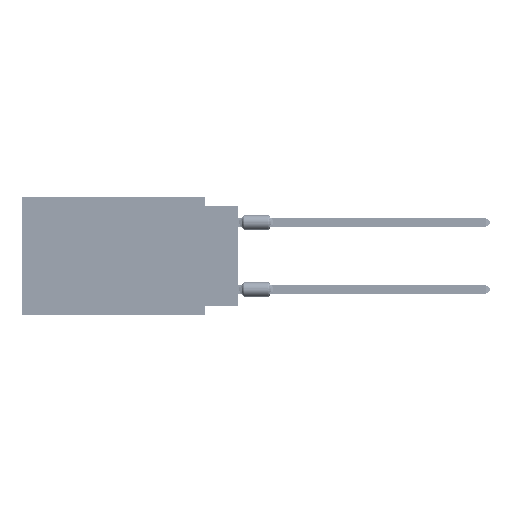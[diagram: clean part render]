
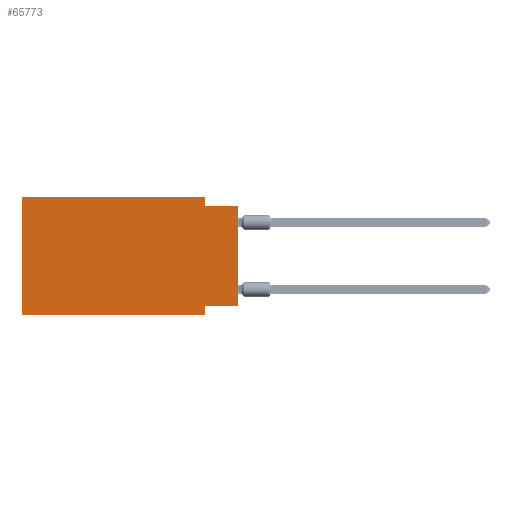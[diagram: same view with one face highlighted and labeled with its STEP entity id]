
A CAD part, left-side view. The second image highlights one B-rep face of the part: STEP entity #65773.
In plain terms, the highlighted planar face has unit normal (-1, 0, 0).
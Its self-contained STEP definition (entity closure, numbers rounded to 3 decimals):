
#11 = CARTESIAN_POINT ( 'NONE',  ( 0., 0., -0.635 ) ) ;
#284 = VERTEX_POINT ( 'NONE', #22249 ) ;
#1347 = DIRECTION ( 'NONE',  ( 1., 0., 0. ) ) ;
#1733 = LINE ( 'NONE', #33577, #5530 ) ;
#3929 = CARTESIAN_POINT ( 'NONE',  ( 0., 2.54, -0.635 ) ) ;
#5530 = VECTOR ( 'NONE', #74538, 1000. ) ;
#5900 = ORIENTED_EDGE ( 'NONE', *, *, #55489, .T. ) ;
#6079 = ORIENTED_EDGE ( 'NONE', *, *, #68950, .F. ) ;
#7489 = VECTOR ( 'NONE', #74238, 1000. ) ;
#7572 = LINE ( 'NONE', #34146, #7489 ) ;
#8371 = LINE ( 'NONE', #22303, #59228 ) ;
#11328 = VECTOR ( 'NONE', #56638, 1000. ) ;
#14348 = VERTEX_POINT ( 'NONE', #56754 ) ;
#15757 = DIRECTION ( 'NONE',  ( 0., -1., 0. ) ) ;
#15805 = CARTESIAN_POINT ( 'NONE',  ( 0., 16.383, 0. ) ) ;
#18344 = LINE ( 'NONE', #57554, #56484 ) ;
#18844 = EDGE_CURVE ( 'NONE', #57992, #76201, #7572, .T. ) ;
#20351 = VECTOR ( 'NONE', #59810, 1000. ) ;
#22249 = CARTESIAN_POINT ( 'NONE',  ( 0., 16.383, 0. ) ) ;
#22303 = CARTESIAN_POINT ( 'NONE',  ( 0., 16.383, 0. ) ) ;
#23098 = LINE ( 'NONE', #49666, #11328 ) ;
#23633 = LINE ( 'NONE', #15805, #83268 ) ;
#24822 = EDGE_CURVE ( 'NONE', #14348, #79552, #18344, .T. ) ;
#27155 = EDGE_CURVE ( 'NONE', #57992, #284, #23633, .T. ) ;
#32731 = EDGE_CURVE ( 'NONE', #65692, #35897, #23098, .T. ) ;
#33174 = FACE_OUTER_BOUND ( 'NONE', #43064, .T. ) ;
#33577 = CARTESIAN_POINT ( 'NONE',  ( 0., 2.54, -8.89 ) ) ;
#34146 = CARTESIAN_POINT ( 'NONE',  ( 0., 16.383, -8.89 ) ) ;
#35132 = ORIENTED_EDGE ( 'NONE', *, *, #53036, .F. ) ;
#35801 = ORIENTED_EDGE ( 'NONE', *, *, #59684, .F. ) ;
#35838 = DIRECTION ( 'NONE',  ( 0., 0., 1. ) ) ;
#35897 = VERTEX_POINT ( 'NONE', #3929 ) ;
#36611 = CARTESIAN_POINT ( 'NONE',  ( 0., 2.54, -8.255 ) ) ;
#37577 = ORIENTED_EDGE ( 'NONE', *, *, #32731, .F. ) ;
#39212 = DIRECTION ( 'NONE',  ( 0., -1., 0. ) ) ;
#40916 = VECTOR ( 'NONE', #39212, 1000. ) ;
#43064 = EDGE_LOOP ( 'NONE', ( #5900, #6079, #37577, #35132, #73326, #68299, #35801, #71181 ) ) ;
#45422 = CARTESIAN_POINT ( 'NONE',  ( 0., 0., 0. ) ) ;
#49666 = CARTESIAN_POINT ( 'NONE',  ( 0., 2.54, 0. ) ) ;
#50329 = CARTESIAN_POINT ( 'NONE',  ( 0., 16.383, -8.89 ) ) ;
#51965 = LINE ( 'NONE', #45422, #20351 ) ;
#53036 = EDGE_CURVE ( 'NONE', #284, #65692, #8371, .T. ) ;
#53158 = LINE ( 'NONE', #11, #40916 ) ;
#53300 = AXIS2_PLACEMENT_3D ( 'NONE', #74561, #1347, #81098 ) ;
#55489 = EDGE_CURVE ( 'NONE', #14348, #77654, #51965, .T. ) ;
#56484 = VECTOR ( 'NONE', #57132, 1000. ) ;
#56638 = DIRECTION ( 'NONE',  ( 0., 0., -1. ) ) ;
#56754 = CARTESIAN_POINT ( 'NONE',  ( 0., 0., -8.255 ) ) ;
#57132 = DIRECTION ( 'NONE',  ( 0., 1., 0. ) ) ;
#57554 = CARTESIAN_POINT ( 'NONE',  ( 0., 0., -8.255 ) ) ;
#57992 = VERTEX_POINT ( 'NONE', #50329 ) ;
#59228 = VECTOR ( 'NONE', #15757, 1000. ) ;
#59684 = EDGE_CURVE ( 'NONE', #79552, #76201, #1733, .T. ) ;
#59810 = DIRECTION ( 'NONE',  ( 0., 0., 1. ) ) ;
#64144 = CARTESIAN_POINT ( 'NONE',  ( 0., 2.54, 0. ) ) ;
#64306 = CARTESIAN_POINT ( 'NONE',  ( 0., 2.54, -8.89 ) ) ;
#65692 = VERTEX_POINT ( 'NONE', #64144 ) ;
#65773 = ADVANCED_FACE ( 'NONE', ( #33174 ), #85949, .F. ) ;
#68299 = ORIENTED_EDGE ( 'NONE', *, *, #18844, .T. ) ;
#68950 = EDGE_CURVE ( 'NONE', #35897, #77654, #53158, .T. ) ;
#71181 = ORIENTED_EDGE ( 'NONE', *, *, #24822, .F. ) ;
#73326 = ORIENTED_EDGE ( 'NONE', *, *, #27155, .F. ) ;
#74238 = DIRECTION ( 'NONE',  ( 0., -1., 0. ) ) ;
#74538 = DIRECTION ( 'NONE',  ( 0., 0., -1. ) ) ;
#74561 = CARTESIAN_POINT ( 'NONE',  ( 0., 16.383, 0. ) ) ;
#76033 = CARTESIAN_POINT ( 'NONE',  ( 0., 0., -0.635 ) ) ;
#76201 = VERTEX_POINT ( 'NONE', #64306 ) ;
#77654 = VERTEX_POINT ( 'NONE', #76033 ) ;
#79552 = VERTEX_POINT ( 'NONE', #36611 ) ;
#81098 = DIRECTION ( 'NONE',  ( 0., 0., -1. ) ) ;
#83268 = VECTOR ( 'NONE', #35838, 1000. ) ;
#85949 = PLANE ( 'NONE',  #53300 ) ;
